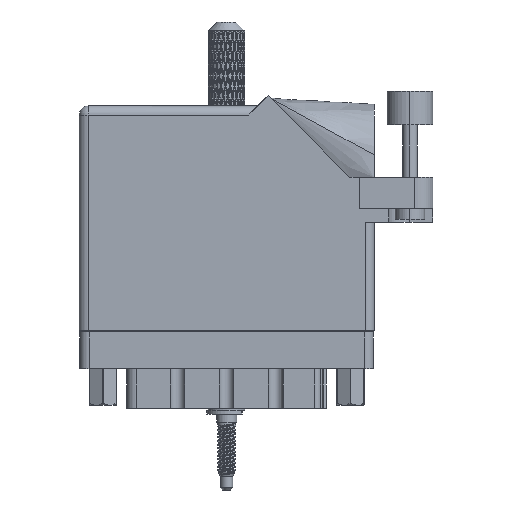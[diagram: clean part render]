
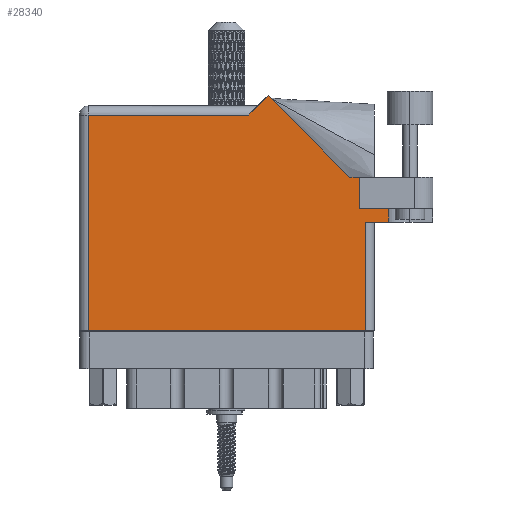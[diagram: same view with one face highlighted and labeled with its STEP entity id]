
A CAD part, front view. The second image highlights one B-rep face of the part: STEP entity #28340.
In plain terms, the highlighted face is planar.
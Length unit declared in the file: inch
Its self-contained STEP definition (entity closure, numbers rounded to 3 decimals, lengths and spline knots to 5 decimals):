
#565 = VERTEX_POINT ( 'NONE', #18837 ) ;
#3885 = CARTESIAN_POINT ( 'NONE',  ( 1.948, 0., 0. ) ) ;
#5156 = ORIENTED_EDGE ( 'NONE', *, *, #94794, .T. ) ;
#7093 = CARTESIAN_POINT ( 'NONE',  ( 0.062, 0., 0. ) ) ;
#7710 = VERTEX_POINT ( 'NONE', #92410 ) ;
#9658 = DIRECTION ( 'NONE',  ( -1., 0., 0. ) ) ;
#10624 = DIRECTION ( 'NONE',  ( 1., 0., 0. ) ) ;
#10818 = EDGE_CURVE ( 'NONE', #90533, #108450, #52570, .T. ) ;
#15092 = LINE ( 'NONE', #71807, #69283 ) ;
#16548 = ORIENTED_EDGE ( 'NONE', *, *, #63203, .T. ) ;
#16559 = CARTESIAN_POINT ( 'NONE',  ( 1.84442, 1.044, 0. ) ) ;
#17356 = CARTESIAN_POINT ( 'NONE',  ( 2.1115, 0.737, 0. ) ) ;
#18482 = EDGE_CURVE ( 'NONE', #48881, #25114, #42987, .T. ) ;
#18509 = LINE ( 'NONE', #79905, #55021 ) ;
#18837 = CARTESIAN_POINT ( 'NONE',  ( 0.062, 0., 0. ) ) ;
#19891 = ORIENTED_EDGE ( 'NONE', *, *, #18482, .T. ) ;
#20078 = CARTESIAN_POINT ( 'NONE',  ( 1.28771, 1.60071, 0. ) ) ;
#21468 = PLANE ( 'NONE',  #85757 ) ;
#24936 = ORIENTED_EDGE ( 'NONE', *, *, #28594, .T. ) ;
#25114 = VERTEX_POINT ( 'NONE', #28104 ) ;
#25623 = DIRECTION ( 'NONE',  ( -0.707, 0.707, 0. ) ) ;
#25823 = CARTESIAN_POINT ( 'NONE',  ( 1.91, 0.831, 0. ) ) ;
#26043 = DIRECTION ( 'NONE',  ( -1., 0., 0. ) ) ;
#28104 = CARTESIAN_POINT ( 'NONE',  ( 1.91, 1.044, 0. ) ) ;
#28340 = ADVANCED_FACE ( 'NONE', ( #73940 ), #21468, .F. ) ;
#28594 = EDGE_CURVE ( 'NONE', #7710, #79084, #18509, .T. ) ;
#29670 = DIRECTION ( 'NONE',  ( 1., 0., 0. ) ) ;
#35547 = EDGE_CURVE ( 'NONE', #110921, #38010, #110993, .T. ) ;
#36180 = VECTOR ( 'NONE', #86103, 39.37008 ) ;
#37563 = ORIENTED_EDGE ( 'NONE', *, *, #69839, .F. ) ;
#38010 = VERTEX_POINT ( 'NONE', #87094 ) ;
#40002 = ORIENTED_EDGE ( 'NONE', *, *, #35547, .T. ) ;
#40916 = VECTOR ( 'NONE', #44115, 39.37008 ) ;
#42033 = VECTOR ( 'NONE', #29670, 39.37008 ) ;
#42644 = ORIENTED_EDGE ( 'NONE', *, *, #81096, .T. ) ;
#42987 = LINE ( 'NONE', #65201, #46946 ) ;
#44115 = DIRECTION ( 'NONE',  ( -0.707, -0.707, 0. ) ) ;
#44408 = EDGE_CURVE ( 'NONE', #82126, #79084, #15092, .T. ) ;
#44414 = VECTOR ( 'NONE', #25623, 39.37008 ) ;
#44753 = LINE ( 'NONE', #56076, #42033 ) ;
#46946 = VECTOR ( 'NONE', #90439, 39.37008 ) ;
#47580 = DIRECTION ( 'NONE',  ( 0., 0., -1. ) ) ;
#47621 = LINE ( 'NONE', #61892, #40916 ) ;
#48881 = VERTEX_POINT ( 'NONE', #72210 ) ;
#52570 = LINE ( 'NONE', #16559, #44414 ) ;
#53883 = CARTESIAN_POINT ( 'NONE',  ( 1.948, 0.737, 0. ) ) ;
#53989 = CARTESIAN_POINT ( 'NONE',  ( 1.84442, 1.044, 0. ) ) ;
#55021 = VECTOR ( 'NONE', #10624, 39.37008 ) ;
#55166 = VECTOR ( 'NONE', #102543, 39.37008 ) ;
#56076 = CARTESIAN_POINT ( 'NONE',  ( 0., 0., 0. ) ) ;
#56226 = DIRECTION ( 'NONE',  ( 0., -1., 0. ) ) ;
#57682 = VECTOR ( 'NONE', #98817, 39.37008 ) ;
#58860 = CARTESIAN_POINT ( 'NONE',  ( 2.1115, 0.831, 0. ) ) ;
#59250 = EDGE_CURVE ( 'NONE', #100662, #7710, #83416, .T. ) ;
#61892 = CARTESIAN_POINT ( 'NONE',  ( 1.217, 1.53, 0. ) ) ;
#62311 = CARTESIAN_POINT ( 'NONE',  ( 0., 1.468, 0. ) ) ;
#63203 = EDGE_CURVE ( 'NONE', #108450, #110921, #47621, .T. ) ;
#63325 = CARTESIAN_POINT ( 'NONE',  ( 1.155, 1.468, 0. ) ) ;
#65201 = CARTESIAN_POINT ( 'NONE',  ( 1.91, 0.831, 0. ) ) ;
#69283 = VECTOR ( 'NONE', #56226, 39.37008 ) ;
#69839 = EDGE_CURVE ( 'NONE', #48881, #82126, #97185, .T. ) ;
#71307 = LINE ( 'NONE', #7093, #36180 ) ;
#71807 = CARTESIAN_POINT ( 'NONE',  ( 2.1115, 1.16177, 0. ) ) ;
#72210 = CARTESIAN_POINT ( 'NONE',  ( 1.91, 0.831, 0. ) ) ;
#72502 = DIRECTION ( 'NONE',  ( -1., 0., 0. ) ) ;
#73940 = FACE_OUTER_BOUND ( 'NONE', #110333, .T. ) ;
#76203 = ORIENTED_EDGE ( 'NONE', *, *, #59250, .T. ) ;
#77205 = ORIENTED_EDGE ( 'NONE', *, *, #90975, .T. ) ;
#78396 = ORIENTED_EDGE ( 'NONE', *, *, #44408, .F. ) ;
#79084 = VERTEX_POINT ( 'NONE', #17356 ) ;
#79905 = CARTESIAN_POINT ( 'NONE',  ( 2.01, 0.737, 0. ) ) ;
#80733 = VECTOR ( 'NONE', #26043, 39.37008 ) ;
#81096 = EDGE_CURVE ( 'NONE', #25114, #90533, #83468, .T. ) ;
#82126 = VERTEX_POINT ( 'NONE', #58860 ) ;
#83416 = LINE ( 'NONE', #53883, #57682 ) ;
#83468 = LINE ( 'NONE', #94430, #80733 ) ;
#85757 = AXIS2_PLACEMENT_3D ( 'NONE', #90601, #47580, #72502 ) ;
#86103 = DIRECTION ( 'NONE',  ( 0., -1., 0. ) ) ;
#87094 = CARTESIAN_POINT ( 'NONE',  ( 0.062, 1.468, 0. ) ) ;
#90439 = DIRECTION ( 'NONE',  ( 0., 1., 0. ) ) ;
#90533 = VERTEX_POINT ( 'NONE', #53989 ) ;
#90601 = CARTESIAN_POINT ( 'NONE',  ( 0., 1.53, 0. ) ) ;
#90975 = EDGE_CURVE ( 'NONE', #565, #100662, #44753, .T. ) ;
#92410 = CARTESIAN_POINT ( 'NONE',  ( 1.948, 0.737, 0. ) ) ;
#94430 = CARTESIAN_POINT ( 'NONE',  ( 2.41, 1.044, 0. ) ) ;
#94794 = EDGE_CURVE ( 'NONE', #38010, #565, #71307, .T. ) ;
#96452 = ORIENTED_EDGE ( 'NONE', *, *, #10818, .T. ) ;
#97185 = LINE ( 'NONE', #25823, #55166 ) ;
#98817 = DIRECTION ( 'NONE',  ( 0., 1., 0. ) ) ;
#100662 = VERTEX_POINT ( 'NONE', #3885 ) ;
#102543 = DIRECTION ( 'NONE',  ( 1., 0., 0. ) ) ;
#102804 = VECTOR ( 'NONE', #9658, 39.37008 ) ;
#108450 = VERTEX_POINT ( 'NONE', #20078 ) ;
#110333 = EDGE_LOOP ( 'NONE', ( #77205, #76203, #24936, #78396, #37563, #19891, #42644, #96452, #16548, #40002, #5156 ) ) ;
#110921 = VERTEX_POINT ( 'NONE', #63325 ) ;
#110993 = LINE ( 'NONE', #62311, #102804 ) ;
